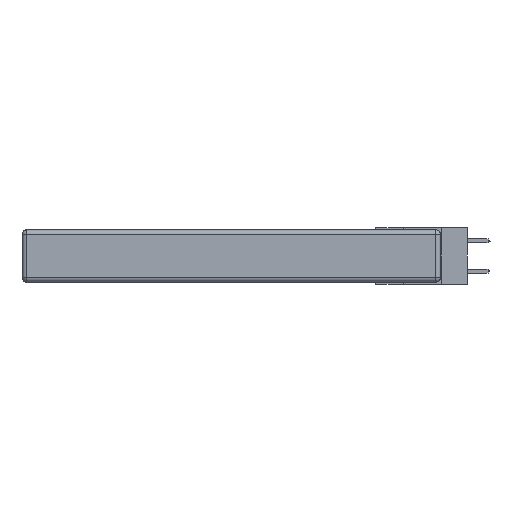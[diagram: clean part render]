
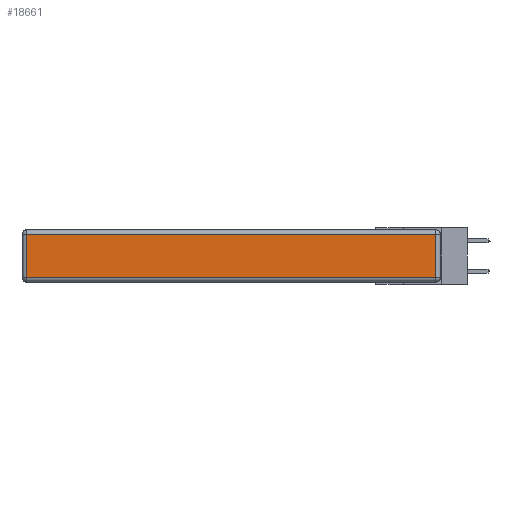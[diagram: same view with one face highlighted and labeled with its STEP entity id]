
A CAD part, left-side view. The second image highlights one B-rep face of the part: STEP entity #18661.
In plain terms, the highlighted planar face has unit normal (-1, 0, 0).
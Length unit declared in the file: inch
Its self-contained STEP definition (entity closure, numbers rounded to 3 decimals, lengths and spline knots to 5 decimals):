
#718 = EDGE_LOOP ( 'NONE', ( #15488, #17296, #12706, #2096 ) ) ;
#1695 = CARTESIAN_POINT ( 'NONE',  ( 0., 2.72, -0.03 ) ) ;
#2096 = ORIENTED_EDGE ( 'NONE', *, *, #6883, .T. ) ;
#2219 = VECTOR ( 'NONE', #6767, 39.37008 ) ;
#2751 = CARTESIAN_POINT ( 'NONE',  ( 0., 0.03, -0.03 ) ) ;
#3185 = PLANE ( 'NONE',  #7774 ) ;
#3253 = CARTESIAN_POINT ( 'NONE',  ( 0., 2.75, -0.03 ) ) ;
#3430 = CARTESIAN_POINT ( 'NONE',  ( 0., 0.03, -0.343 ) ) ;
#4495 = LINE ( 'NONE', #15699, #16934 ) ;
#4542 = EDGE_CURVE ( 'NONE', #10825, #10352, #5023, .T. ) ;
#5023 = LINE ( 'NONE', #3253, #15430 ) ;
#5735 = DIRECTION ( 'NONE',  ( 0., 1., 0. ) ) ;
#5896 = VECTOR ( 'NONE', #9281, 39.37008 ) ;
#6767 = DIRECTION ( 'NONE',  ( 0., -1., 0. ) ) ;
#6883 = EDGE_CURVE ( 'NONE', #10352, #8575, #4495, .T. ) ;
#7181 = LINE ( 'NONE', #16991, #2219 ) ;
#7774 = AXIS2_PLACEMENT_3D ( 'NONE', #10111, #16021, #13156 ) ;
#8575 = VERTEX_POINT ( 'NONE', #12985 ) ;
#9281 = DIRECTION ( 'NONE',  ( 0., 0., 1. ) ) ;
#10076 = FACE_OUTER_BOUND ( 'NONE', #718, .T. ) ;
#10111 = CARTESIAN_POINT ( 'NONE',  ( 0., 0., -0.343 ) ) ;
#10352 = VERTEX_POINT ( 'NONE', #1695 ) ;
#10653 = VERTEX_POINT ( 'NONE', #15129 ) ;
#10825 = VERTEX_POINT ( 'NONE', #2751 ) ;
#12489 = EDGE_CURVE ( 'NONE', #10653, #10825, #16953, .T. ) ;
#12706 = ORIENTED_EDGE ( 'NONE', *, *, #4542, .T. ) ;
#12985 = CARTESIAN_POINT ( 'NONE',  ( 0., 2.72, -0.313 ) ) ;
#13156 = DIRECTION ( 'NONE',  ( 0., 0., 1. ) ) ;
#15129 = CARTESIAN_POINT ( 'NONE',  ( 0., 0.03, -0.313 ) ) ;
#15430 = VECTOR ( 'NONE', #5735, 39.37008 ) ;
#15488 = ORIENTED_EDGE ( 'NONE', *, *, #18079, .T. ) ;
#15699 = CARTESIAN_POINT ( 'NONE',  ( 0., 2.72, -0.343 ) ) ;
#16021 = DIRECTION ( 'NONE',  ( -1., 0., 0. ) ) ;
#16934 = VECTOR ( 'NONE', #17074, 39.37008 ) ;
#16953 = LINE ( 'NONE', #3430, #5896 ) ;
#16991 = CARTESIAN_POINT ( 'NONE',  ( 0., 0., -0.313 ) ) ;
#17074 = DIRECTION ( 'NONE',  ( 0., 0., -1. ) ) ;
#17296 = ORIENTED_EDGE ( 'NONE', *, *, #12489, .T. ) ;
#18079 = EDGE_CURVE ( 'NONE', #8575, #10653, #7181, .T. ) ;
#18661 = ADVANCED_FACE ( 'NONE', ( #10076 ), #3185, .T. ) ;
